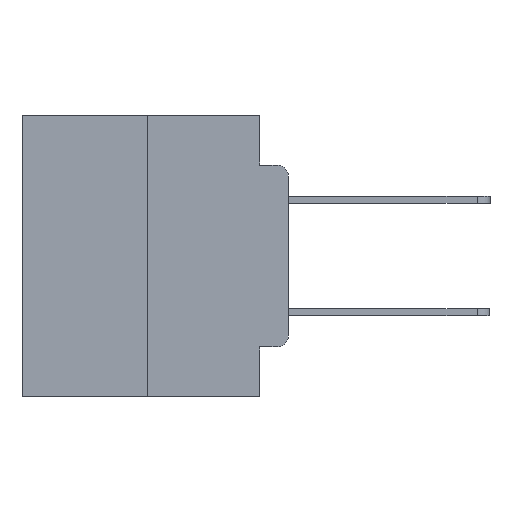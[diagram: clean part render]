
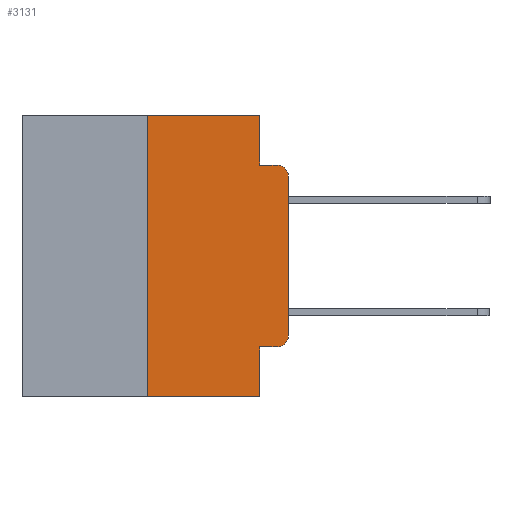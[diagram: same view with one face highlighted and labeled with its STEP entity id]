
A CAD part, left-side view. The second image highlights one B-rep face of the part: STEP entity #3131.
In plain terms, the highlighted planar face has unit normal (-1, 0, 0).
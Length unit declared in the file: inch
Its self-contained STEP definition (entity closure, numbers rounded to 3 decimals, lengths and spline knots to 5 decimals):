
#5 = DIRECTION ( 'NONE',  ( 0., -1., 0. ) ) ;
#1282 = CARTESIAN_POINT ( 'NONE',  ( 0., 0.02, -0.0885 ) ) ;
#1599 = CARTESIAN_POINT ( 'NONE',  ( 0., 0.02, -0.4115 ) ) ;
#1829 = AXIS2_PLACEMENT_3D ( 'NONE', #23517, #11498, #25404 ) ;
#2502 = VECTOR ( 'NONE', #6853, 39.37008 ) ;
#2594 = CARTESIAN_POINT ( 'NONE',  ( 0., 0.051, -0.4115 ) ) ;
#2783 = CARTESIAN_POINT ( 'NONE',  ( 0., 0.051, 0. ) ) ;
#3074 = CARTESIAN_POINT ( 'NONE',  ( 0., 0.051, -0.0885 ) ) ;
#3131 = ADVANCED_FACE ( 'NONE', ( #18387 ), #13160, .F. ) ;
#3268 = VECTOR ( 'NONE', #17017, 39.37008 ) ;
#3890 = VERTEX_POINT ( 'NONE', #1599 ) ;
#3927 = LINE ( 'NONE', #15008, #3268 ) ;
#4064 = ORIENTED_EDGE ( 'NONE', *, *, #15315, .F. ) ;
#4341 = CARTESIAN_POINT ( 'NONE',  ( 0., 0.051, -0.5 ) ) ;
#4702 = CARTESIAN_POINT ( 'NONE',  ( 0., 0.473, -0.5 ) ) ;
#4916 = CARTESIAN_POINT ( 'NONE',  ( 0., 0.473, 0. ) ) ;
#4992 = CARTESIAN_POINT ( 'NONE',  ( 0., 0.051, -0.4115 ) ) ;
#5142 = VECTOR ( 'NONE', #8896, 39.37008 ) ;
#5498 = VERTEX_POINT ( 'NONE', #3074 ) ;
#6236 = LINE ( 'NONE', #2594, #11663 ) ;
#6853 = DIRECTION ( 'NONE',  ( 0., -1., 0. ) ) ;
#6987 = CIRCLE ( 'NONE', #16903, 0.02 ) ;
#7168 = VERTEX_POINT ( 'NONE', #1282 ) ;
#7273 = DIRECTION ( 'NONE',  ( 0., 0., -1. ) ) ;
#7592 = DIRECTION ( 'NONE',  ( -1., 0., 0. ) ) ;
#7694 = ORIENTED_EDGE ( 'NONE', *, *, #22082, .F. ) ;
#7805 = VERTEX_POINT ( 'NONE', #23595 ) ;
#7907 = VERTEX_POINT ( 'NONE', #19910 ) ;
#8063 = LINE ( 'NONE', #21755, #22881 ) ;
#8232 = EDGE_CURVE ( 'NONE', #7805, #23724, #24106, .T. ) ;
#8664 = ORIENTED_EDGE ( 'NONE', *, *, #11259, .T. ) ;
#8896 = DIRECTION ( 'NONE',  ( 0., -1., 0. ) ) ;
#9128 = VECTOR ( 'NONE', #5, 39.37008 ) ;
#10032 = CARTESIAN_POINT ( 'NONE',  ( 0., 0.051, 0. ) ) ;
#10170 = VERTEX_POINT ( 'NONE', #13995 ) ;
#10876 = DIRECTION ( 'NONE',  ( 0., -1., 0. ) ) ;
#11133 = VERTEX_POINT ( 'NONE', #2783 ) ;
#11194 = CIRCLE ( 'NONE', #1829, 0.02 ) ;
#11259 = EDGE_CURVE ( 'NONE', #3890, #10170, #6987, .T. ) ;
#11498 = DIRECTION ( 'NONE',  ( -1., 0., 0. ) ) ;
#11663 = VECTOR ( 'NONE', #10876, 39.37008 ) ;
#11685 = CARTESIAN_POINT ( 'NONE',  ( 0., 0.25, 0. ) ) ;
#12153 = DIRECTION ( 'NONE',  ( 0., 0., -1. ) ) ;
#12611 = EDGE_CURVE ( 'NONE', #24665, #3890, #6236, .T. ) ;
#12743 = LINE ( 'NONE', #11685, #22211 ) ;
#13160 = PLANE ( 'NONE',  #23311 ) ;
#13708 = DIRECTION ( 'NONE',  ( 0., 0., 1. ) ) ;
#13949 = EDGE_CURVE ( 'NONE', #24665, #23724, #8063, .T. ) ;
#13995 = CARTESIAN_POINT ( 'NONE',  ( 0., 0., -0.3915 ) ) ;
#14501 = LINE ( 'NONE', #20393, #9128 ) ;
#14679 = CARTESIAN_POINT ( 'NONE',  ( 0., 0., -0.1085 ) ) ;
#15008 = CARTESIAN_POINT ( 'NONE',  ( 0., 0., 0. ) ) ;
#15315 = EDGE_CURVE ( 'NONE', #7805, #7907, #12743, .T. ) ;
#16129 = LINE ( 'NONE', #10032, #20882 ) ;
#16547 = ORIENTED_EDGE ( 'NONE', *, *, #23381, .T. ) ;
#16668 = EDGE_CURVE ( 'NONE', #11133, #5498, #16129, .T. ) ;
#16862 = ORIENTED_EDGE ( 'NONE', *, *, #13949, .F. ) ;
#16903 = AXIS2_PLACEMENT_3D ( 'NONE', #19640, #7592, #21739 ) ;
#17017 = DIRECTION ( 'NONE',  ( 0., 0., 1. ) ) ;
#17367 = EDGE_CURVE ( 'NONE', #7907, #11133, #14501, .T. ) ;
#18083 = ORIENTED_EDGE ( 'NONE', *, *, #12611, .T. ) ;
#18387 = FACE_OUTER_BOUND ( 'NONE', #19475, .T. ) ;
#18836 = VERTEX_POINT ( 'NONE', #14679 ) ;
#19021 = ORIENTED_EDGE ( 'NONE', *, *, #16668, .F. ) ;
#19475 = EDGE_LOOP ( 'NONE', ( #25784, #16547, #7694, #19021, #19660, #4064, #26095, #16862, #18083, #8664 ) ) ;
#19640 = CARTESIAN_POINT ( 'NONE',  ( 0., 0.02, -0.3915 ) ) ;
#19660 = ORIENTED_EDGE ( 'NONE', *, *, #17367, .F. ) ;
#19910 = CARTESIAN_POINT ( 'NONE',  ( 0., 0.25, 0. ) ) ;
#20393 = CARTESIAN_POINT ( 'NONE',  ( 0., 0.473, 0. ) ) ;
#20882 = VECTOR ( 'NONE', #12153, 39.37008 ) ;
#21375 = LINE ( 'NONE', #24883, #5142 ) ;
#21739 = DIRECTION ( 'NONE',  ( 0., 0., -1. ) ) ;
#21755 = CARTESIAN_POINT ( 'NONE',  ( 0., 0.051, 0. ) ) ;
#22082 = EDGE_CURVE ( 'NONE', #5498, #7168, #21375, .T. ) ;
#22211 = VECTOR ( 'NONE', #13708, 39.37008 ) ;
#22881 = VECTOR ( 'NONE', #23689, 39.37008 ) ;
#23311 = AXIS2_PLACEMENT_3D ( 'NONE', #4916, #25260, #7273 ) ;
#23381 = EDGE_CURVE ( 'NONE', #18836, #7168, #11194, .T. ) ;
#23517 = CARTESIAN_POINT ( 'NONE',  ( 0., 0.02, -0.1085 ) ) ;
#23595 = CARTESIAN_POINT ( 'NONE',  ( 0., 0.25, -0.5 ) ) ;
#23689 = DIRECTION ( 'NONE',  ( 0., 0., -1. ) ) ;
#23724 = VERTEX_POINT ( 'NONE', #4341 ) ;
#24106 = LINE ( 'NONE', #4702, #2502 ) ;
#24665 = VERTEX_POINT ( 'NONE', #4992 ) ;
#24883 = CARTESIAN_POINT ( 'NONE',  ( 0., 0.051, -0.0885 ) ) ;
#25260 = DIRECTION ( 'NONE',  ( 1., 0., 0. ) ) ;
#25404 = DIRECTION ( 'NONE',  ( 0., 0., -1. ) ) ;
#25784 = ORIENTED_EDGE ( 'NONE', *, *, #25902, .T. ) ;
#25902 = EDGE_CURVE ( 'NONE', #10170, #18836, #3927, .T. ) ;
#26095 = ORIENTED_EDGE ( 'NONE', *, *, #8232, .T. ) ;
